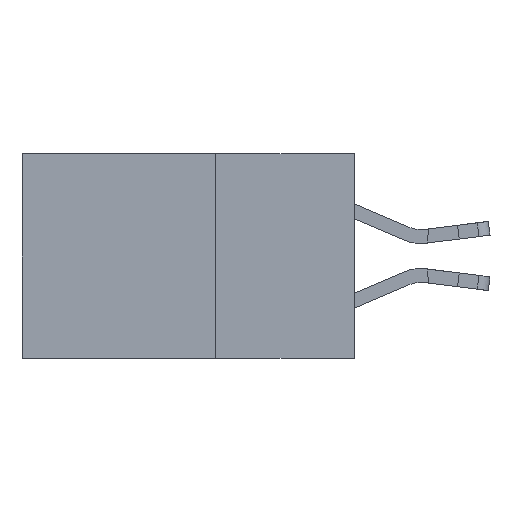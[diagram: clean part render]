
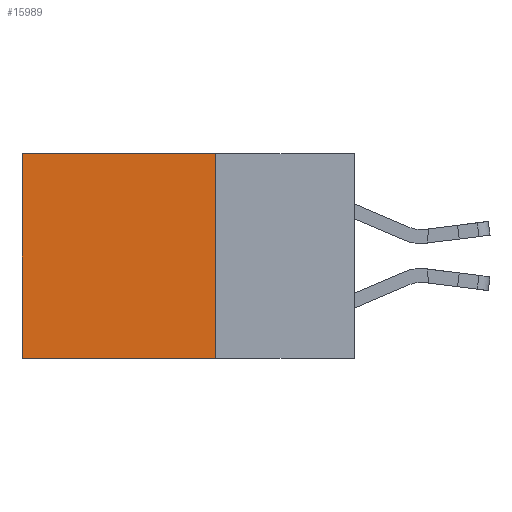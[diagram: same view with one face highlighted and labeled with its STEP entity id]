
A CAD part, left-side view. The second image highlights one B-rep face of the part: STEP entity #15989.
In plain terms, the highlighted planar face has unit normal (-1, 0, 0).
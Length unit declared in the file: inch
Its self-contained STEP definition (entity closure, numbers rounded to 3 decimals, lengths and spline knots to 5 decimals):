
#11 = CARTESIAN_POINT ( 'NONE',  ( 0.2615, 0.25, -0.37 ) ) ;
#25 = VECTOR ( 'NONE', #9968, 39.37008 ) ;
#348 = CARTESIAN_POINT ( 'NONE',  ( 0.2615, 0.6, 0. ) ) ;
#1759 = DIRECTION ( 'NONE',  ( 0., 0., -1. ) ) ;
#2459 = CARTESIAN_POINT ( 'NONE',  ( 0.2615, 0.25, -0.37 ) ) ;
#3595 = DIRECTION ( 'NONE',  ( 0., 0., -1. ) ) ;
#3999 = ORIENTED_EDGE ( 'NONE', *, *, #19123, .F. ) ;
#4098 = ORIENTED_EDGE ( 'NONE', *, *, #15584, .F. ) ;
#5160 = FACE_OUTER_BOUND ( 'NONE', #7516, .T. ) ;
#5381 = CARTESIAN_POINT ( 'NONE',  ( 0.2615, 0.6, -0.37 ) ) ;
#6650 = DIRECTION ( 'NONE',  ( 0., 1., 0. ) ) ;
#6990 = VECTOR ( 'NONE', #8588, 39.37008 ) ;
#7222 = EDGE_CURVE ( 'NONE', #12404, #17590, #18778, .T. ) ;
#7516 = EDGE_LOOP ( 'NONE', ( #17862, #4098, #3999, #15949 ) ) ;
#7689 = LINE ( 'NONE', #10814, #18527 ) ;
#8588 = DIRECTION ( 'NONE',  ( 0., 1., 0. ) ) ;
#9008 = VERTEX_POINT ( 'NONE', #10616 ) ;
#9159 = DIRECTION ( 'NONE',  ( 1., 0., 0. ) ) ;
#9968 = DIRECTION ( 'NONE',  ( 0., 0., -1. ) ) ;
#10164 = LINE ( 'NONE', #2459, #6990 ) ;
#10363 = VERTEX_POINT ( 'NONE', #11 ) ;
#10415 = VECTOR ( 'NONE', #6650, 39.37008 ) ;
#10616 = CARTESIAN_POINT ( 'NONE',  ( 0.2615, 0.25, 0. ) ) ;
#10814 = CARTESIAN_POINT ( 'NONE',  ( 0.2615, 0.25, -0.37 ) ) ;
#12404 = VERTEX_POINT ( 'NONE', #348 ) ;
#12589 = CARTESIAN_POINT ( 'NONE',  ( 0.2615, 0.25, 0. ) ) ;
#13214 = EDGE_CURVE ( 'NONE', #9008, #12404, #18692, .T. ) ;
#13222 = CARTESIAN_POINT ( 'NONE',  ( 0.2615, 0.6, -0.37 ) ) ;
#14788 = AXIS2_PLACEMENT_3D ( 'NONE', #18174, #9159, #1759 ) ;
#15584 = EDGE_CURVE ( 'NONE', #10363, #17590, #10164, .T. ) ;
#15949 = ORIENTED_EDGE ( 'NONE', *, *, #13214, .T. ) ;
#15989 = ADVANCED_FACE ( 'NONE', ( #5160 ), #17081, .F. ) ;
#17081 = PLANE ( 'NONE',  #14788 ) ;
#17590 = VERTEX_POINT ( 'NONE', #13222 ) ;
#17862 = ORIENTED_EDGE ( 'NONE', *, *, #7222, .T. ) ;
#18174 = CARTESIAN_POINT ( 'NONE',  ( 0.2615, 0.25, -0.37 ) ) ;
#18527 = VECTOR ( 'NONE', #3595, 39.37008 ) ;
#18692 = LINE ( 'NONE', #12589, #10415 ) ;
#18778 = LINE ( 'NONE', #5381, #25 ) ;
#19123 = EDGE_CURVE ( 'NONE', #9008, #10363, #7689, .T. ) ;
